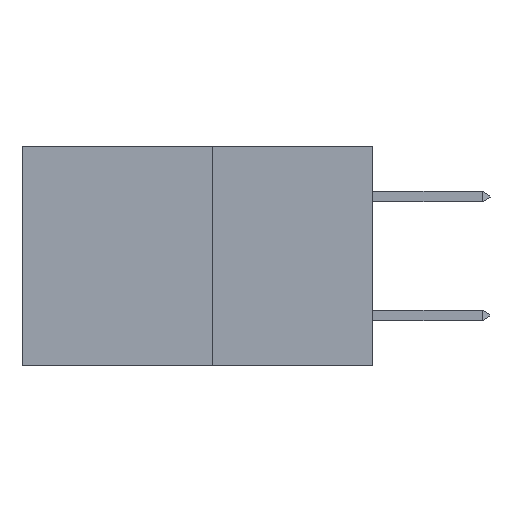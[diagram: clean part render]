
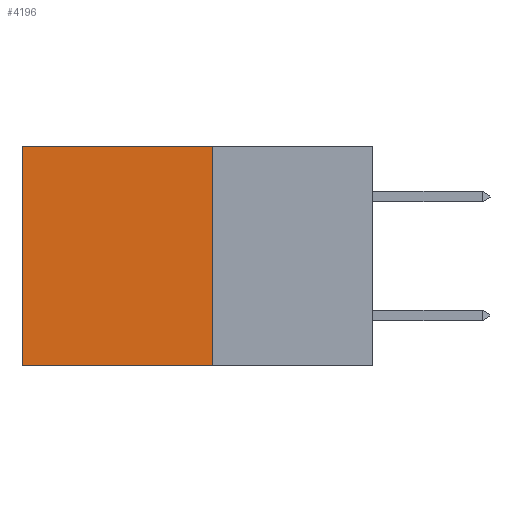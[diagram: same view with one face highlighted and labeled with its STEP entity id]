
A CAD part, left-side view. The second image highlights one B-rep face of the part: STEP entity #4196.
In plain terms, the highlighted planar face has unit normal (-1, 0, 0).
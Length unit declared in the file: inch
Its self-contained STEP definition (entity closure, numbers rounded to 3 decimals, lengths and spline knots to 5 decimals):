
#387 = LINE ( 'NONE', #6228, #7781 ) ;
#485 = AXIS2_PLACEMENT_3D ( 'NONE', #1727, #1545, #1536 ) ;
#599 = ORIENTED_EDGE ( 'NONE', *, *, #8132, .F. ) ;
#665 = ORIENTED_EDGE ( 'NONE', *, *, #2856, .T. ) ;
#718 = VERTEX_POINT ( 'NONE', #2653 ) ;
#937 = VECTOR ( 'NONE', #5295, 39.37008 ) ;
#1070 = ORIENTED_EDGE ( 'NONE', *, *, #7127, .T. ) ;
#1536 = DIRECTION ( 'NONE',  ( 0., 0., -1. ) ) ;
#1545 = DIRECTION ( 'NONE',  ( 1., 0., 0. ) ) ;
#1585 = PLANE ( 'NONE',  #485 ) ;
#1727 = CARTESIAN_POINT ( 'NONE',  ( 0.277, 0.27, -0.37 ) ) ;
#1781 = ORIENTED_EDGE ( 'NONE', *, *, #2253, .F. ) ;
#2253 = EDGE_CURVE ( 'NONE', #4810, #718, #387, .T. ) ;
#2653 = CARTESIAN_POINT ( 'NONE',  ( 0.277, 0.59, -0.37 ) ) ;
#2856 = EDGE_CURVE ( 'NONE', #7208, #5820, #6312, .T. ) ;
#3919 = CARTESIAN_POINT ( 'NONE',  ( 0.277, 0.27, 0. ) ) ;
#4058 = CARTESIAN_POINT ( 'NONE',  ( 0.277, 0.27, -0.37 ) ) ;
#4196 = ADVANCED_FACE ( 'NONE', ( #7954 ), #1585, .F. ) ;
#4316 = VECTOR ( 'NONE', #7963, 39.37008 ) ;
#4684 = VECTOR ( 'NONE', #6017, 39.37008 ) ;
#4810 = VERTEX_POINT ( 'NONE', #4058 ) ;
#4900 = CARTESIAN_POINT ( 'NONE',  ( 0.277, 0.27, 0. ) ) ;
#5295 = DIRECTION ( 'NONE',  ( 0., 0., -1. ) ) ;
#5510 = CARTESIAN_POINT ( 'NONE',  ( 0.277, 0.59, -0.37 ) ) ;
#5820 = VERTEX_POINT ( 'NONE', #8319 ) ;
#6017 = DIRECTION ( 'NONE',  ( 0., 0., -1. ) ) ;
#6072 = CARTESIAN_POINT ( 'NONE',  ( 0.277, 0.27, -0.37 ) ) ;
#6228 = CARTESIAN_POINT ( 'NONE',  ( 0.277, 0.27, -0.37 ) ) ;
#6312 = LINE ( 'NONE', #4900, #4316 ) ;
#6458 = LINE ( 'NONE', #6072, #4684 ) ;
#6692 = LINE ( 'NONE', #5510, #937 ) ;
#7127 = EDGE_CURVE ( 'NONE', #5820, #718, #6692, .T. ) ;
#7208 = VERTEX_POINT ( 'NONE', #3919 ) ;
#7393 = EDGE_LOOP ( 'NONE', ( #1070, #1781, #599, #665 ) ) ;
#7781 = VECTOR ( 'NONE', #8129, 39.37008 ) ;
#7954 = FACE_OUTER_BOUND ( 'NONE', #7393, .T. ) ;
#7963 = DIRECTION ( 'NONE',  ( 0., 1., 0. ) ) ;
#8129 = DIRECTION ( 'NONE',  ( 0., 1., 0. ) ) ;
#8132 = EDGE_CURVE ( 'NONE', #7208, #4810, #6458, .T. ) ;
#8319 = CARTESIAN_POINT ( 'NONE',  ( 0.277, 0.59, 0. ) ) ;
